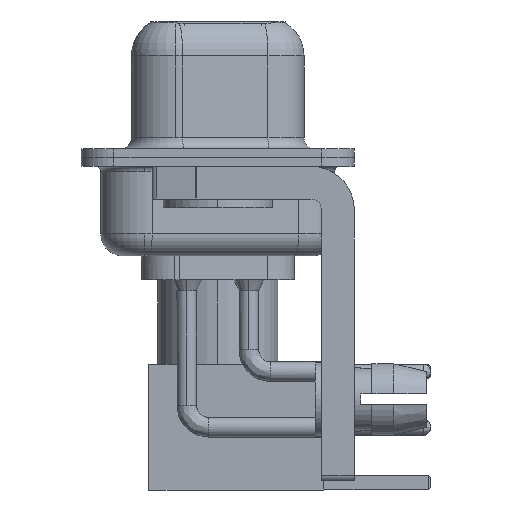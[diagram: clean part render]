
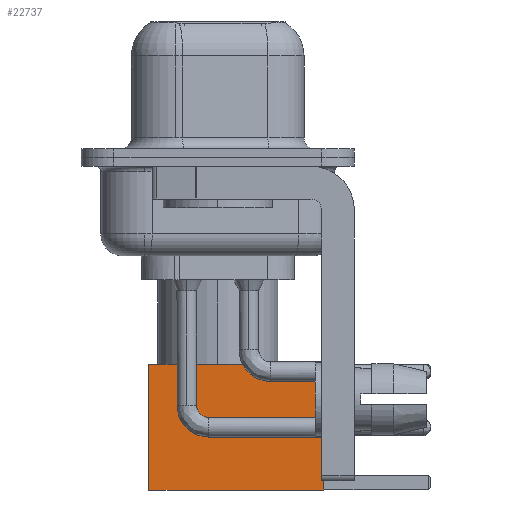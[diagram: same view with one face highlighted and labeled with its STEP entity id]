
A CAD part, left-side view. The second image highlights one B-rep face of the part: STEP entity #22737.
In plain terms, the highlighted face is planar.
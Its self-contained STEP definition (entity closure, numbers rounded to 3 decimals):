
#274 = VECTOR ( 'NONE', #5231, 1000. ) ;
#501 = CARTESIAN_POINT ( 'NONE',  ( 2.875, 2.875, 0. ) ) ;
#1247 = VERTEX_POINT ( 'NONE', #21394 ) ;
#1718 = CARTESIAN_POINT ( 'NONE',  ( -2.875, 2.875, 0. ) ) ;
#3490 = CARTESIAN_POINT ( 'NONE',  ( 0., 2.875, 8. ) ) ;
#4065 = LINE ( 'NONE', #501, #4320 ) ;
#4309 = DIRECTION ( 'NONE',  ( 0., 0., -1. ) ) ;
#4320 = VECTOR ( 'NONE', #4309, 1000. ) ;
#5056 = CARTESIAN_POINT ( 'NONE',  ( 2.875, 2.875, 0. ) ) ;
#5231 = DIRECTION ( 'NONE',  ( -1., 0., 0. ) ) ;
#6934 = VECTOR ( 'NONE', #9474, 1000. ) ;
#6952 = EDGE_CURVE ( 'NONE', #24187, #1247, #8990, .T. ) ;
#8207 = ORIENTED_EDGE ( 'NONE', *, *, #22423, .T. ) ;
#8990 = LINE ( 'NONE', #3490, #6934 ) ;
#9302 = VERTEX_POINT ( 'NONE', #5056 ) ;
#9474 = DIRECTION ( 'NONE',  ( -1., 0., 0. ) ) ;
#9488 = EDGE_CURVE ( 'NONE', #24187, #9302, #4065, .T. ) ;
#9791 = VERTEX_POINT ( 'NONE', #1718 ) ;
#10107 = CARTESIAN_POINT ( 'NONE',  ( 2.875, 2.875, 0. ) ) ;
#10225 = PLANE ( 'NONE',  #20232 ) ;
#10280 = EDGE_CURVE ( 'NONE', #1247, #9791, #15034, .T. ) ;
#11348 = ORIENTED_EDGE ( 'NONE', *, *, #6952, .F. ) ;
#11553 = CARTESIAN_POINT ( 'NONE',  ( 2.875, 2.875, 8. ) ) ;
#15034 = LINE ( 'NONE', #16864, #18430 ) ;
#15237 = ORIENTED_EDGE ( 'NONE', *, *, #9488, .T. ) ;
#16384 = DIRECTION ( 'NONE',  ( 0., 0., -1. ) ) ;
#16864 = CARTESIAN_POINT ( 'NONE',  ( -2.875, 2.875, 0. ) ) ;
#18430 = VECTOR ( 'NONE', #16384, 1000. ) ;
#19653 = DIRECTION ( 'NONE',  ( 0., 0., 1. ) ) ;
#19697 = EDGE_LOOP ( 'NONE', ( #15237, #8207, #24071, #11348 ) ) ;
#19775 = FACE_OUTER_BOUND ( 'NONE', #19697, .T. ) ;
#20232 = AXIS2_PLACEMENT_3D ( 'NONE', #10107, #23338, #19653 ) ;
#21394 = CARTESIAN_POINT ( 'NONE',  ( -2.875, 2.875, 8. ) ) ;
#21999 = LINE ( 'NONE', #23959, #274 ) ;
#22423 = EDGE_CURVE ( 'NONE', #9302, #9791, #21999, .T. ) ;
#22737 = ADVANCED_FACE ( 'NONE', ( #19775 ), #10225, .T. ) ;
#23338 = DIRECTION ( 'NONE',  ( 0., 1., 0. ) ) ;
#23959 = CARTESIAN_POINT ( 'NONE',  ( 0., 2.875, 0. ) ) ;
#24071 = ORIENTED_EDGE ( 'NONE', *, *, #10280, .F. ) ;
#24187 = VERTEX_POINT ( 'NONE', #11553 ) ;
